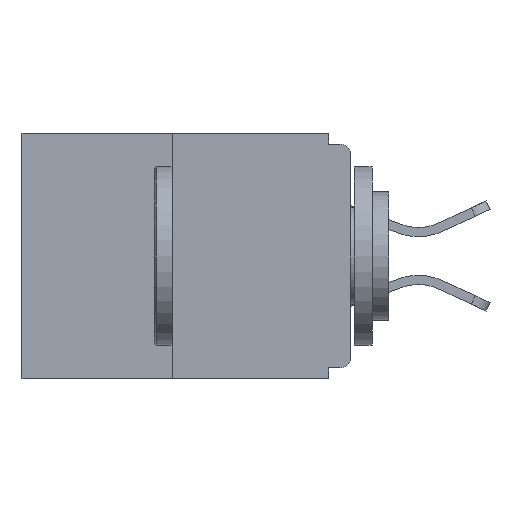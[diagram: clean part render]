
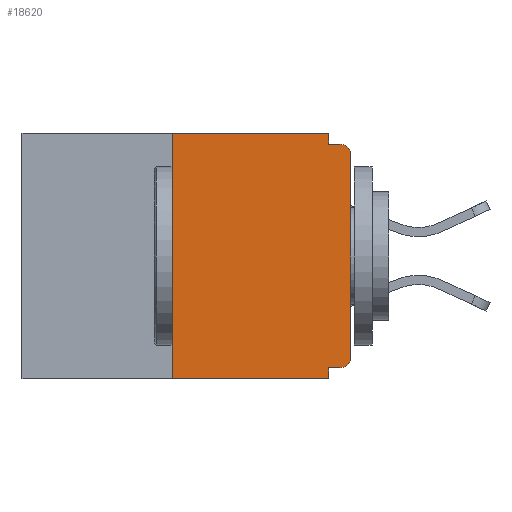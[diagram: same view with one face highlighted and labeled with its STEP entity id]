
A CAD part, left-side view. The second image highlights one B-rep face of the part: STEP entity #18620.
In plain terms, the highlighted planar face has unit normal (-1, 0, 0).
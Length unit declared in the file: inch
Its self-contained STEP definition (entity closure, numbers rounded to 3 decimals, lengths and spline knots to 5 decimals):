
#185 = DIRECTION ( 'NONE',  ( -1., 0., 0. ) ) ;
#360 = DIRECTION ( 'NONE',  ( 1., 0., 0. ) ) ;
#472 = CARTESIAN_POINT ( 'NONE',  ( 0., 0.46, 0. ) ) ;
#659 = VECTOR ( 'NONE', #17407, 39.37008 ) ;
#717 = ORIENTED_EDGE ( 'NONE', *, *, #19927, .T. ) ;
#1531 = ORIENTED_EDGE ( 'NONE', *, *, #15454, .F. ) ;
#1630 = CARTESIAN_POINT ( 'NONE',  ( 0., 0.015, -0.015 ) ) ;
#1681 = LINE ( 'NONE', #14003, #659 ) ;
#1902 = CARTESIAN_POINT ( 'NONE',  ( 0., 0., -0.328 ) ) ;
#1980 = ORIENTED_EDGE ( 'NONE', *, *, #2747, .F. ) ;
#1996 = DIRECTION ( 'NONE',  ( 0., 0., -1. ) ) ;
#2747 = EDGE_CURVE ( 'NONE', #9334, #7795, #16698, .T. ) ;
#3113 = VERTEX_POINT ( 'NONE', #6863 ) ;
#3458 = ORIENTED_EDGE ( 'NONE', *, *, #4924, .T. ) ;
#3835 = VERTEX_POINT ( 'NONE', #12391 ) ;
#3866 = EDGE_CURVE ( 'NONE', #4729, #3113, #16679, .T. ) ;
#3872 = VECTOR ( 'NONE', #15104, 39.37008 ) ;
#4248 = CARTESIAN_POINT ( 'NONE',  ( 0., 0.015, -0.328 ) ) ;
#4482 = ORIENTED_EDGE ( 'NONE', *, *, #6099, .T. ) ;
#4729 = VERTEX_POINT ( 'NONE', #20083 ) ;
#4737 = EDGE_CURVE ( 'NONE', #4729, #8582, #8651, .T. ) ;
#4924 = EDGE_CURVE ( 'NONE', #3835, #9666, #15105, .T. ) ;
#5080 = ORIENTED_EDGE ( 'NONE', *, *, #16637, .F. ) ;
#5150 = CARTESIAN_POINT ( 'NONE',  ( 0., 0.46, 0. ) ) ;
#5251 = ORIENTED_EDGE ( 'NONE', *, *, #4737, .T. ) ;
#5420 = CIRCLE ( 'NONE', #17413, 0.015 ) ;
#5942 = ORIENTED_EDGE ( 'NONE', *, *, #3866, .F. ) ;
#6099 = EDGE_CURVE ( 'NONE', #6877, #3835, #10073, .T. ) ;
#6383 = AXIS2_PLACEMENT_3D ( 'NONE', #6658, #185, #11467 ) ;
#6658 = CARTESIAN_POINT ( 'NONE',  ( 0., 0.015, -0.03 ) ) ;
#6778 = PLANE ( 'NONE',  #7902 ) ;
#6832 = VECTOR ( 'NONE', #19581, 39.37008 ) ;
#6863 = CARTESIAN_POINT ( 'NONE',  ( 0., 0.25, 0. ) ) ;
#6866 = VECTOR ( 'NONE', #15236, 39.37008 ) ;
#6877 = VERTEX_POINT ( 'NONE', #8988 ) ;
#7052 = DIRECTION ( 'NONE',  ( 0., 0., 1. ) ) ;
#7111 = DIRECTION ( 'NONE',  ( 0., -1., 0. ) ) ;
#7269 = CARTESIAN_POINT ( 'NONE',  ( 0., 0.031, -0.328 ) ) ;
#7345 = VECTOR ( 'NONE', #19948, 39.37008 ) ;
#7795 = VERTEX_POINT ( 'NONE', #7269 ) ;
#7902 = AXIS2_PLACEMENT_3D ( 'NONE', #5150, #360, #1996 ) ;
#8075 = VECTOR ( 'NONE', #7111, 39.37008 ) ;
#8365 = DIRECTION ( 'NONE',  ( 0., 1., 0. ) ) ;
#8582 = VERTEX_POINT ( 'NONE', #20122 ) ;
#8651 = LINE ( 'NONE', #18697, #3872 ) ;
#8988 = CARTESIAN_POINT ( 'NONE',  ( 0., 0., -0.313 ) ) ;
#9219 = DIRECTION ( 'NONE',  ( -1., 0., 0. ) ) ;
#9326 = EDGE_LOOP ( 'NONE', ( #1531, #5942, #5251, #11065, #1980, #717, #4482, #3458, #5080, #18256 ) ) ;
#9334 = VERTEX_POINT ( 'NONE', #4248 ) ;
#9666 = VERTEX_POINT ( 'NONE', #1630 ) ;
#10073 = LINE ( 'NONE', #17959, #6832 ) ;
#10250 = CARTESIAN_POINT ( 'NONE',  ( 0., 0.031, -0.015 ) ) ;
#10448 = CARTESIAN_POINT ( 'NONE',  ( 0., 0., -0.015 ) ) ;
#11065 = ORIENTED_EDGE ( 'NONE', *, *, #15864, .F. ) ;
#11258 = VERTEX_POINT ( 'NONE', #18432 ) ;
#11467 = DIRECTION ( 'NONE',  ( 0., 0., -1. ) ) ;
#11980 = EDGE_CURVE ( 'NONE', #11258, #20378, #1681, .T. ) ;
#12391 = CARTESIAN_POINT ( 'NONE',  ( 0., 0., -0.03 ) ) ;
#12466 = CARTESIAN_POINT ( 'NONE',  ( 0., 0.015, -0.313 ) ) ;
#13182 = FACE_OUTER_BOUND ( 'NONE', #9326, .T. ) ;
#13670 = VECTOR ( 'NONE', #8365, 39.37008 ) ;
#14003 = CARTESIAN_POINT ( 'NONE',  ( 0., 0.031, 0. ) ) ;
#15061 = CARTESIAN_POINT ( 'NONE',  ( 0., 0.031, -0.343 ) ) ;
#15104 = DIRECTION ( 'NONE',  ( 0., -1., 0. ) ) ;
#15105 = CIRCLE ( 'NONE', #6383, 0.015 ) ;
#15236 = DIRECTION ( 'NONE',  ( 0., -1., 0. ) ) ;
#15337 = LINE ( 'NONE', #472, #6866 ) ;
#15454 = EDGE_CURVE ( 'NONE', #3113, #11258, #15337, .T. ) ;
#15864 = EDGE_CURVE ( 'NONE', #7795, #8582, #16323, .T. ) ;
#16323 = LINE ( 'NONE', #15061, #7345 ) ;
#16637 = EDGE_CURVE ( 'NONE', #20378, #9666, #20623, .T. ) ;
#16679 = LINE ( 'NONE', #16686, #18484 ) ;
#16686 = CARTESIAN_POINT ( 'NONE',  ( 0., 0.25, 0. ) ) ;
#16698 = LINE ( 'NONE', #1902, #13670 ) ;
#17407 = DIRECTION ( 'NONE',  ( 0., 0., -1. ) ) ;
#17413 = AXIS2_PLACEMENT_3D ( 'NONE', #12466, #9219, #20387 ) ;
#17959 = CARTESIAN_POINT ( 'NONE',  ( 0., 0., 0. ) ) ;
#18256 = ORIENTED_EDGE ( 'NONE', *, *, #11980, .F. ) ;
#18432 = CARTESIAN_POINT ( 'NONE',  ( 0., 0.031, 0. ) ) ;
#18484 = VECTOR ( 'NONE', #7052, 39.37008 ) ;
#18620 = ADVANCED_FACE ( 'NONE', ( #13182 ), #6778, .F. ) ;
#18697 = CARTESIAN_POINT ( 'NONE',  ( 0., 0.46, -0.343 ) ) ;
#19581 = DIRECTION ( 'NONE',  ( 0., 0., 1. ) ) ;
#19927 = EDGE_CURVE ( 'NONE', #9334, #6877, #5420, .T. ) ;
#19948 = DIRECTION ( 'NONE',  ( 0., 0., -1. ) ) ;
#20083 = CARTESIAN_POINT ( 'NONE',  ( 0., 0.25, -0.343 ) ) ;
#20122 = CARTESIAN_POINT ( 'NONE',  ( 0., 0.031, -0.343 ) ) ;
#20378 = VERTEX_POINT ( 'NONE', #10250 ) ;
#20387 = DIRECTION ( 'NONE',  ( 0., 0., -1. ) ) ;
#20623 = LINE ( 'NONE', #10448, #8075 ) ;
